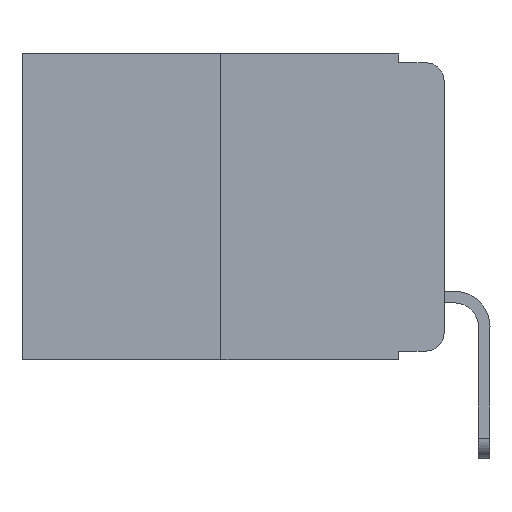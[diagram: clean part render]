
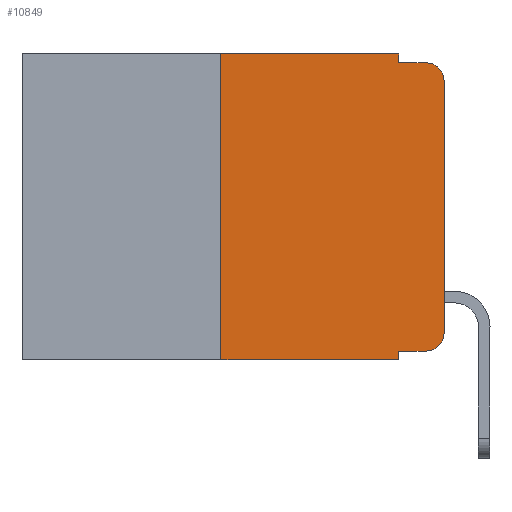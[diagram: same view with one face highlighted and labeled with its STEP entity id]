
A CAD part, left-side view. The second image highlights one B-rep face of the part: STEP entity #10849.
In plain terms, the highlighted planar face has unit normal (-1, 0, 0).
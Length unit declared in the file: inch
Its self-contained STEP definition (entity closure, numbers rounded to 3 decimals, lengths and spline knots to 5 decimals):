
#157 = ORIENTED_EDGE ( 'NONE', *, *, #7385, .F. ) ;
#804 = DIRECTION ( 'NONE',  ( -1., 0., 0. ) ) ;
#846 = VERTEX_POINT ( 'NONE', #16035 ) ;
#1076 = CARTESIAN_POINT ( 'NONE',  ( 0., 0.051, 0. ) ) ;
#1110 = EDGE_CURVE ( 'NONE', #7390, #9212, #13433, .T. ) ;
#1150 = VERTEX_POINT ( 'NONE', #17334 ) ;
#1223 = CIRCLE ( 'NONE', #10465, 0.02 ) ;
#1514 = CARTESIAN_POINT ( 'NONE',  ( 0., 0.02, -0.03 ) ) ;
#2044 = LINE ( 'NONE', #22537, #6027 ) ;
#2644 = VERTEX_POINT ( 'NONE', #23120 ) ;
#3573 = VERTEX_POINT ( 'NONE', #22480 ) ;
#3903 = ORIENTED_EDGE ( 'NONE', *, *, #12531, .F. ) ;
#4050 = CARTESIAN_POINT ( 'NONE',  ( 0., 0.25, 0. ) ) ;
#4219 = ORIENTED_EDGE ( 'NONE', *, *, #7802, .T. ) ;
#4311 = DIRECTION ( 'NONE',  ( 0., 0., -1. ) ) ;
#4476 = DIRECTION ( 'NONE',  ( 1., 0., 0. ) ) ;
#4569 = EDGE_CURVE ( 'NONE', #7390, #15888, #14752, .T. ) ;
#4643 = ORIENTED_EDGE ( 'NONE', *, *, #10020, .F. ) ;
#4694 = CARTESIAN_POINT ( 'NONE',  ( 0., 0.02, -0.333 ) ) ;
#5339 = DIRECTION ( 'NONE',  ( 0., 0., 1. ) ) ;
#5723 = VECTOR ( 'NONE', #20715, 39.37008 ) ;
#5803 = DIRECTION ( 'NONE',  ( 0., -1., 0. ) ) ;
#5982 = CARTESIAN_POINT ( 'NONE',  ( 0., 0.473, -0.343 ) ) ;
#6027 = VECTOR ( 'NONE', #6316, 39.37008 ) ;
#6209 = CARTESIAN_POINT ( 'NONE',  ( 0., 0.25, -0.343 ) ) ;
#6316 = DIRECTION ( 'NONE',  ( 0., -1., 0. ) ) ;
#6339 = DIRECTION ( 'NONE',  ( 0., -1., 0. ) ) ;
#7228 = CARTESIAN_POINT ( 'NONE',  ( 0., 0., 0. ) ) ;
#7385 = EDGE_CURVE ( 'NONE', #846, #2644, #2044, .T. ) ;
#7390 = VERTEX_POINT ( 'NONE', #9735 ) ;
#7802 = EDGE_CURVE ( 'NONE', #7836, #9212, #14854, .T. ) ;
#7836 = VERTEX_POINT ( 'NONE', #6209 ) ;
#8202 = VECTOR ( 'NONE', #13708, 39.37008 ) ;
#8764 = LINE ( 'NONE', #1076, #8202 ) ;
#8822 = EDGE_LOOP ( 'NONE', ( #15926, #17187, #11113, #4643, #157, #3903, #4219, #14915, #17615, #9152 ) ) ;
#9152 = ORIENTED_EDGE ( 'NONE', *, *, #21062, .T. ) ;
#9212 = VERTEX_POINT ( 'NONE', #18927 ) ;
#9221 = AXIS2_PLACEMENT_3D ( 'NONE', #13693, #4476, #4311 ) ;
#9647 = DIRECTION ( 'NONE',  ( 0., 0., -1. ) ) ;
#9735 = CARTESIAN_POINT ( 'NONE',  ( 0., 0.051, -0.333 ) ) ;
#10020 = EDGE_CURVE ( 'NONE', #2644, #13336, #8764, .T. ) ;
#10074 = VECTOR ( 'NONE', #5339, 39.37008 ) ;
#10465 = AXIS2_PLACEMENT_3D ( 'NONE', #17159, #804, #9647 ) ;
#10561 = CIRCLE ( 'NONE', #20095, 0.02 ) ;
#10849 = ADVANCED_FACE ( 'NONE', ( #21011 ), #17238, .F. ) ;
#10924 = LINE ( 'NONE', #7228, #10074 ) ;
#11113 = ORIENTED_EDGE ( 'NONE', *, *, #22135, .F. ) ;
#11275 = DIRECTION ( 'NONE',  ( 0., 0., 1. ) ) ;
#12531 = EDGE_CURVE ( 'NONE', #7836, #846, #19983, .T. ) ;
#12651 = DIRECTION ( 'NONE',  ( 0., 0., -1. ) ) ;
#13336 = VERTEX_POINT ( 'NONE', #21819 ) ;
#13388 = DIRECTION ( 'NONE',  ( 0., 0., -1. ) ) ;
#13433 = LINE ( 'NONE', #22533, #22336 ) ;
#13693 = CARTESIAN_POINT ( 'NONE',  ( 0., 0.473, 0. ) ) ;
#13708 = DIRECTION ( 'NONE',  ( 0., 0., -1. ) ) ;
#14248 = DIRECTION ( 'NONE',  ( -1., 0., 0. ) ) ;
#14500 = VERTEX_POINT ( 'NONE', #16273 ) ;
#14752 = LINE ( 'NONE', #18413, #18205 ) ;
#14854 = LINE ( 'NONE', #5982, #5723 ) ;
#14915 = ORIENTED_EDGE ( 'NONE', *, *, #1110, .F. ) ;
#15888 = VERTEX_POINT ( 'NONE', #4694 ) ;
#15926 = ORIENTED_EDGE ( 'NONE', *, *, #20027, .T. ) ;
#16018 = LINE ( 'NONE', #21109, #23437 ) ;
#16035 = CARTESIAN_POINT ( 'NONE',  ( 0., 0.25, 0. ) ) ;
#16273 = CARTESIAN_POINT ( 'NONE',  ( 0., 0.02, -0.01 ) ) ;
#17159 = CARTESIAN_POINT ( 'NONE',  ( 0., 0.02, -0.313 ) ) ;
#17187 = ORIENTED_EDGE ( 'NONE', *, *, #21939, .T. ) ;
#17238 = PLANE ( 'NONE',  #9221 ) ;
#17334 = CARTESIAN_POINT ( 'NONE',  ( 0., 0., -0.03 ) ) ;
#17615 = ORIENTED_EDGE ( 'NONE', *, *, #4569, .T. ) ;
#18205 = VECTOR ( 'NONE', #5803, 39.37008 ) ;
#18282 = VECTOR ( 'NONE', #11275, 39.37008 ) ;
#18413 = CARTESIAN_POINT ( 'NONE',  ( 0., 0.051, -0.333 ) ) ;
#18927 = CARTESIAN_POINT ( 'NONE',  ( 0., 0.051, -0.343 ) ) ;
#19983 = LINE ( 'NONE', #4050, #18282 ) ;
#20027 = EDGE_CURVE ( 'NONE', #3573, #1150, #10924, .T. ) ;
#20095 = AXIS2_PLACEMENT_3D ( 'NONE', #1514, #14248, #12651 ) ;
#20715 = DIRECTION ( 'NONE',  ( 0., -1., 0. ) ) ;
#21011 = FACE_OUTER_BOUND ( 'NONE', #8822, .T. ) ;
#21062 = EDGE_CURVE ( 'NONE', #15888, #3573, #1223, .T. ) ;
#21109 = CARTESIAN_POINT ( 'NONE',  ( 0., 0.051, -0.01 ) ) ;
#21819 = CARTESIAN_POINT ( 'NONE',  ( 0., 0.051, -0.01 ) ) ;
#21939 = EDGE_CURVE ( 'NONE', #1150, #14500, #10561, .T. ) ;
#22135 = EDGE_CURVE ( 'NONE', #13336, #14500, #16018, .T. ) ;
#22336 = VECTOR ( 'NONE', #13388, 39.37008 ) ;
#22480 = CARTESIAN_POINT ( 'NONE',  ( 0., 0., -0.313 ) ) ;
#22533 = CARTESIAN_POINT ( 'NONE',  ( 0., 0.051, 0. ) ) ;
#22537 = CARTESIAN_POINT ( 'NONE',  ( 0., 0.473, 0. ) ) ;
#23120 = CARTESIAN_POINT ( 'NONE',  ( 0., 0.051, 0. ) ) ;
#23437 = VECTOR ( 'NONE', #6339, 39.37008 ) ;
